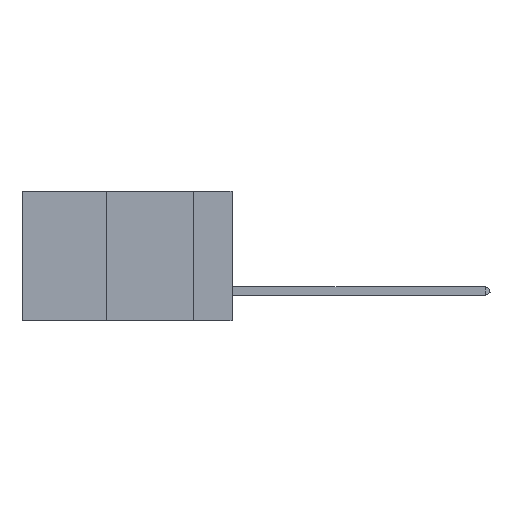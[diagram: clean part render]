
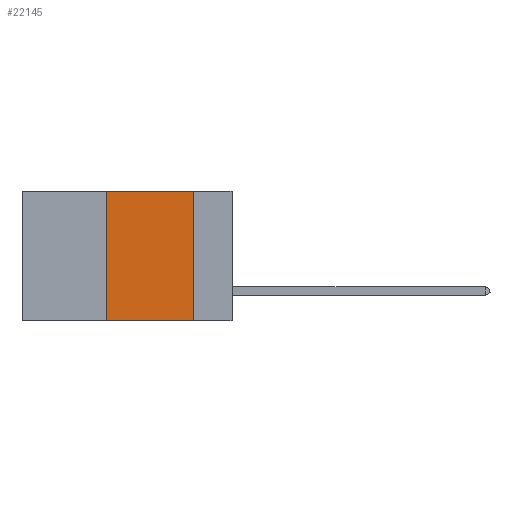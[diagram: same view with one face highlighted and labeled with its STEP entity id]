
A CAD part, left-side view. The second image highlights one B-rep face of the part: STEP entity #22145.
In plain terms, the highlighted planar face has unit normal (-1, 0, 0).
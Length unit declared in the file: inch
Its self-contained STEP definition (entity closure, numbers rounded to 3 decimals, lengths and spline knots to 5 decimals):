
#238 = LINE ( 'NONE', #21033, #4307 ) ;
#486 = ORIENTED_EDGE ( 'NONE', *, *, #19775, .T. ) ;
#3114 = CARTESIAN_POINT ( 'NONE',  ( 0., 0.36, 0. ) ) ;
#3333 = CARTESIAN_POINT ( 'NONE',  ( 0., 0.36, -0.37 ) ) ;
#4307 = VECTOR ( 'NONE', #9910, 39.37008 ) ;
#4873 = VERTEX_POINT ( 'NONE', #7157 ) ;
#5435 = LINE ( 'NONE', #11149, #15667 ) ;
#6322 = VECTOR ( 'NONE', #11245, 39.37008 ) ;
#6723 = DIRECTION ( 'NONE',  ( 0., 0., -1. ) ) ;
#6864 = VECTOR ( 'NONE', #8921, 39.37008 ) ;
#6876 = DIRECTION ( 'NONE',  ( 1., 0., 0. ) ) ;
#7157 = CARTESIAN_POINT ( 'NONE',  ( 0., 0.11, 0. ) ) ;
#8394 = EDGE_CURVE ( 'NONE', #4873, #12051, #238, .T. ) ;
#8413 = ORIENTED_EDGE ( 'NONE', *, *, #20193, .F. ) ;
#8921 = DIRECTION ( 'NONE',  ( 0., 0., 1. ) ) ;
#8962 = LINE ( 'NONE', #3114, #6864 ) ;
#9910 = DIRECTION ( 'NONE',  ( 0., 0., -1. ) ) ;
#10559 = EDGE_LOOP ( 'NONE', ( #16566, #13720, #8413, #486 ) ) ;
#10648 = PLANE ( 'NONE',  #15531 ) ;
#11149 = CARTESIAN_POINT ( 'NONE',  ( 0., 0.6, -0.37 ) ) ;
#11245 = DIRECTION ( 'NONE',  ( 0., -1., 0. ) ) ;
#12051 = VERTEX_POINT ( 'NONE', #14273 ) ;
#13247 = DIRECTION ( 'NONE',  ( 0., -1., 0. ) ) ;
#13698 = VERTEX_POINT ( 'NONE', #16896 ) ;
#13720 = ORIENTED_EDGE ( 'NONE', *, *, #19288, .F. ) ;
#14273 = CARTESIAN_POINT ( 'NONE',  ( 0., 0.11, -0.37 ) ) ;
#15078 = CARTESIAN_POINT ( 'NONE',  ( 0., 0.6, 0. ) ) ;
#15531 = AXIS2_PLACEMENT_3D ( 'NONE', #17865, #6876, #6723 ) ;
#15667 = VECTOR ( 'NONE', #13247, 39.37008 ) ;
#16566 = ORIENTED_EDGE ( 'NONE', *, *, #8394, .F. ) ;
#16896 = CARTESIAN_POINT ( 'NONE',  ( 0., 0.36, 0. ) ) ;
#17681 = LINE ( 'NONE', #15078, #6322 ) ;
#17865 = CARTESIAN_POINT ( 'NONE',  ( 0., 0.6, 0. ) ) ;
#19125 = VERTEX_POINT ( 'NONE', #3333 ) ;
#19288 = EDGE_CURVE ( 'NONE', #13698, #4873, #17681, .T. ) ;
#19775 = EDGE_CURVE ( 'NONE', #19125, #12051, #5435, .T. ) ;
#20193 = EDGE_CURVE ( 'NONE', #19125, #13698, #8962, .T. ) ;
#20796 = FACE_OUTER_BOUND ( 'NONE', #10559, .T. ) ;
#21033 = CARTESIAN_POINT ( 'NONE',  ( 0., 0.11, 0. ) ) ;
#22145 = ADVANCED_FACE ( 'NONE', ( #20796 ), #10648, .F. ) ;
